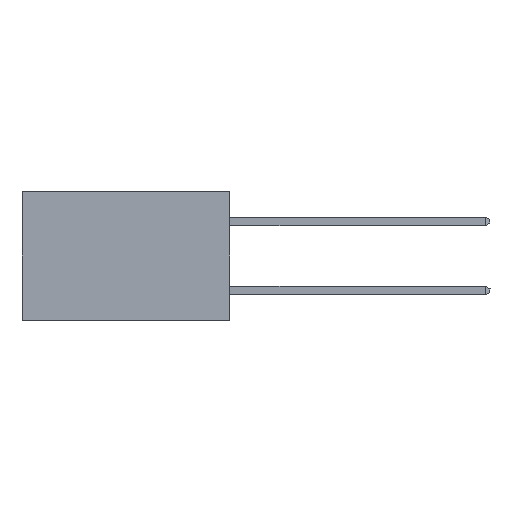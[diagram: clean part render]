
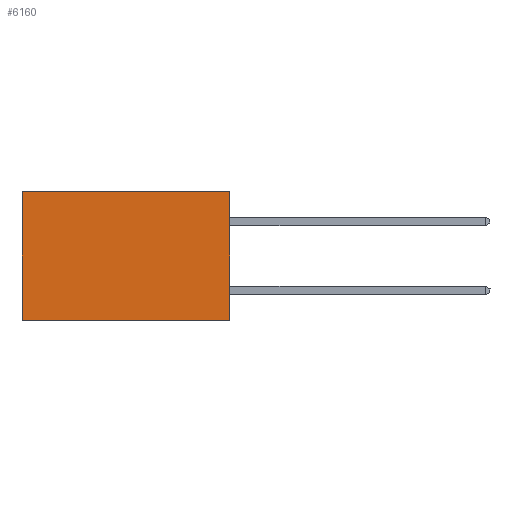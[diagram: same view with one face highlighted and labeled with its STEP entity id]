
A CAD part, left-side view. The second image highlights one B-rep face of the part: STEP entity #6160.
In plain terms, the highlighted planar face has unit normal (-1, 0, 0).
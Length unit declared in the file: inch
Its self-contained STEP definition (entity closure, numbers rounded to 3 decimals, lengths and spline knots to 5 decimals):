
#328 = CARTESIAN_POINT ( 'NONE',  ( 0.298, 0., 0. ) ) ;
#510 = ORIENTED_EDGE ( 'NONE', *, *, #5553, .T. ) ;
#1088 = LINE ( 'NONE', #5661, #10467 ) ;
#1399 = AXIS2_PLACEMENT_3D ( 'NONE', #5844, #14771, #3417 ) ;
#1770 = EDGE_LOOP ( 'NONE', ( #8960, #8732, #3738, #510 ) ) ;
#2929 = EDGE_CURVE ( 'NONE', #6781, #11361, #13282, .T. ) ;
#3417 = DIRECTION ( 'NONE',  ( 0., 0., -1. ) ) ;
#3448 = CARTESIAN_POINT ( 'NONE',  ( 0.298, 0., 0. ) ) ;
#3738 = ORIENTED_EDGE ( 'NONE', *, *, #2929, .F. ) ;
#3740 = VECTOR ( 'NONE', #13794, 39.37008 ) ;
#5006 = CARTESIAN_POINT ( 'NONE',  ( 0.298, 0.6, 0. ) ) ;
#5080 = EDGE_CURVE ( 'NONE', #11361, #12547, #1088, .T. ) ;
#5200 = EDGE_CURVE ( 'NONE', #12274, #12547, #7519, .T. ) ;
#5402 = DIRECTION ( 'NONE',  ( 0., 0., -1. ) ) ;
#5553 = EDGE_CURVE ( 'NONE', #6781, #12274, #11484, .T. ) ;
#5661 = CARTESIAN_POINT ( 'NONE',  ( 0.298, 0., -0.37 ) ) ;
#5844 = CARTESIAN_POINT ( 'NONE',  ( 0.298, 0., 0. ) ) ;
#6160 = ADVANCED_FACE ( 'NONE', ( #11652 ), #16251, .F. ) ;
#6781 = VERTEX_POINT ( 'NONE', #328 ) ;
#7519 = LINE ( 'NONE', #12956, #12666 ) ;
#7986 = CARTESIAN_POINT ( 'NONE',  ( 0.298, 0., 0. ) ) ;
#8262 = CARTESIAN_POINT ( 'NONE',  ( 0.298, 0.6, -0.37 ) ) ;
#8717 = CARTESIAN_POINT ( 'NONE',  ( 0.298, 0., -0.37 ) ) ;
#8732 = ORIENTED_EDGE ( 'NONE', *, *, #5080, .F. ) ;
#8960 = ORIENTED_EDGE ( 'NONE', *, *, #5200, .T. ) ;
#9171 = DIRECTION ( 'NONE',  ( 0., 1., 0. ) ) ;
#9615 = DIRECTION ( 'NONE',  ( 0., 1., 0. ) ) ;
#10467 = VECTOR ( 'NONE', #9615, 39.37008 ) ;
#11361 = VERTEX_POINT ( 'NONE', #8717 ) ;
#11484 = LINE ( 'NONE', #7986, #12065 ) ;
#11652 = FACE_OUTER_BOUND ( 'NONE', #1770, .T. ) ;
#12065 = VECTOR ( 'NONE', #9171, 39.37008 ) ;
#12274 = VERTEX_POINT ( 'NONE', #5006 ) ;
#12547 = VERTEX_POINT ( 'NONE', #8262 ) ;
#12666 = VECTOR ( 'NONE', #5402, 39.37008 ) ;
#12956 = CARTESIAN_POINT ( 'NONE',  ( 0.298, 0.6, 0. ) ) ;
#13282 = LINE ( 'NONE', #3448, #3740 ) ;
#13794 = DIRECTION ( 'NONE',  ( 0., 0., -1. ) ) ;
#14771 = DIRECTION ( 'NONE',  ( 1., 0., 0. ) ) ;
#16251 = PLANE ( 'NONE',  #1399 ) ;
